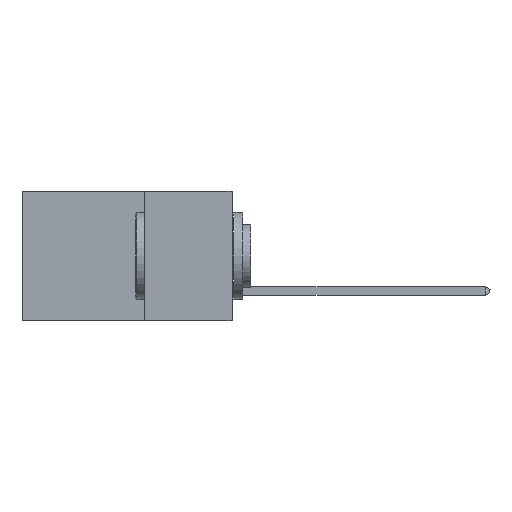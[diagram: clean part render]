
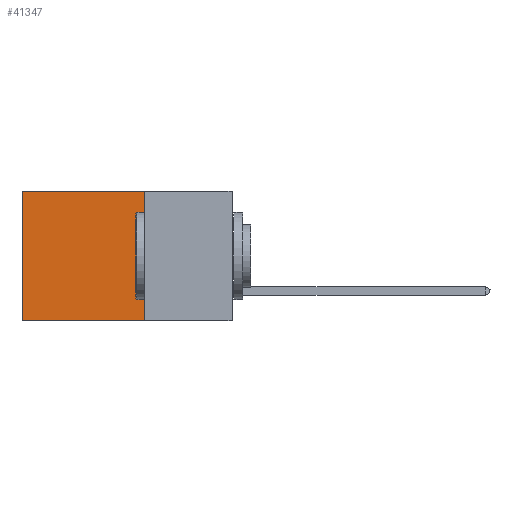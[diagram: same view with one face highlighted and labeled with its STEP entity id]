
A CAD part, left-side view. The second image highlights one B-rep face of the part: STEP entity #41347.
In plain terms, the highlighted planar face has unit normal (-1, 0, 0).
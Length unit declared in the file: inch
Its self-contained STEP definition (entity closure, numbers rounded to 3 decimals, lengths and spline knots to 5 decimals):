
#419 = DIRECTION ( 'NONE',  ( 0., 0., -1. ) ) ;
#2045 = VECTOR ( 'NONE', #41881, 39.37008 ) ;
#2891 = CARTESIAN_POINT ( 'NONE',  ( 0.2875, 0.6, 0. ) ) ;
#4403 = VERTEX_POINT ( 'NONE', #45625 ) ;
#6087 = EDGE_CURVE ( 'NONE', #32546, #23904, #32016, .T. ) ;
#6213 = EDGE_CURVE ( 'NONE', #4403, #23904, #14827, .T. ) ;
#6384 = CARTESIAN_POINT ( 'NONE',  ( 0.2875, 0.25, 0. ) ) ;
#7880 = VERTEX_POINT ( 'NONE', #25541 ) ;
#9541 = VECTOR ( 'NONE', #34356, 39.37008 ) ;
#10313 = EDGE_LOOP ( 'NONE', ( #14947, #33211, #26050, #17060 ) ) ;
#12054 = CARTESIAN_POINT ( 'NONE',  ( 0.2875, 0.25, -0.37 ) ) ;
#12129 = PLANE ( 'NONE',  #13137 ) ;
#13137 = AXIS2_PLACEMENT_3D ( 'NONE', #32873, #22481, #29816 ) ;
#14763 = EDGE_CURVE ( 'NONE', #7880, #4403, #35783, .T. ) ;
#14827 = LINE ( 'NONE', #2891, #20368 ) ;
#14947 = ORIENTED_EDGE ( 'NONE', *, *, #6213, .T. ) ;
#17060 = ORIENTED_EDGE ( 'NONE', *, *, #14763, .T. ) ;
#17434 = EDGE_CURVE ( 'NONE', #7880, #32546, #38349, .T. ) ;
#19763 = CARTESIAN_POINT ( 'NONE',  ( 0.2875, 0.25, 0. ) ) ;
#20368 = VECTOR ( 'NONE', #419, 39.37008 ) ;
#20500 = FACE_OUTER_BOUND ( 'NONE', #10313, .T. ) ;
#22481 = DIRECTION ( 'NONE',  ( 1., 0., 0. ) ) ;
#23904 = VERTEX_POINT ( 'NONE', #27596 ) ;
#25541 = CARTESIAN_POINT ( 'NONE',  ( 0.2875, 0.25, 0. ) ) ;
#26050 = ORIENTED_EDGE ( 'NONE', *, *, #17434, .F. ) ;
#27596 = CARTESIAN_POINT ( 'NONE',  ( 0.2875, 0.6, -0.37 ) ) ;
#29816 = DIRECTION ( 'NONE',  ( 0., 0., -1. ) ) ;
#31138 = DIRECTION ( 'NONE',  ( 0., 1., 0. ) ) ;
#32016 = LINE ( 'NONE', #45130, #2045 ) ;
#32546 = VERTEX_POINT ( 'NONE', #12054 ) ;
#32873 = CARTESIAN_POINT ( 'NONE',  ( 0.2875, 0.25, 0. ) ) ;
#33211 = ORIENTED_EDGE ( 'NONE', *, *, #6087, .F. ) ;
#34136 = VECTOR ( 'NONE', #31138, 39.37008 ) ;
#34356 = DIRECTION ( 'NONE',  ( 0., 0., -1. ) ) ;
#35783 = LINE ( 'NONE', #6384, #34136 ) ;
#38349 = LINE ( 'NONE', #19763, #9541 ) ;
#41347 = ADVANCED_FACE ( 'NONE', ( #20500 ), #12129, .F. ) ;
#41881 = DIRECTION ( 'NONE',  ( 0., 1., 0. ) ) ;
#45130 = CARTESIAN_POINT ( 'NONE',  ( 0.2875, 0.25, -0.37 ) ) ;
#45625 = CARTESIAN_POINT ( 'NONE',  ( 0.2875, 0.6, 0. ) ) ;
